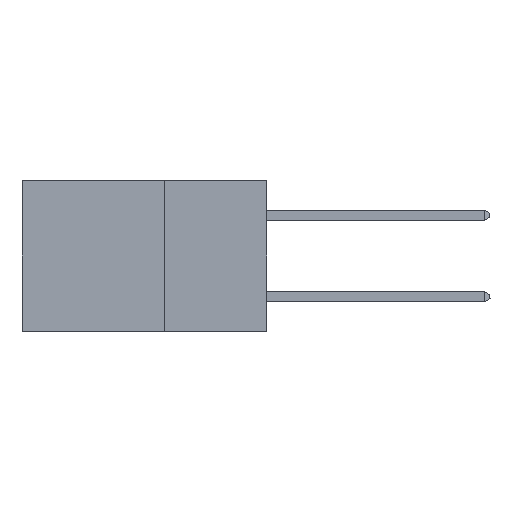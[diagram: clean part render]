
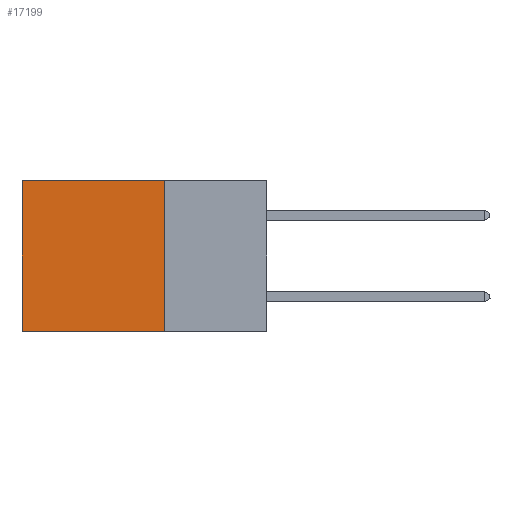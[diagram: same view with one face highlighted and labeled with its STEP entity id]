
A CAD part, left-side view. The second image highlights one B-rep face of the part: STEP entity #17199.
In plain terms, the highlighted planar face has unit normal (-1, 0, 0).
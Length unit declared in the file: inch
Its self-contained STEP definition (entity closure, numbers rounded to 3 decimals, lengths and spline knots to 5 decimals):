
#155 = VERTEX_POINT ( 'NONE', #15002 ) ;
#659 = AXIS2_PLACEMENT_3D ( 'NONE', #4516, #7272, #16826 ) ;
#1121 = EDGE_CURVE ( 'NONE', #13793, #7417, #9360, .T. ) ;
#1685 = ORIENTED_EDGE ( 'NONE', *, *, #1121, .F. ) ;
#1804 = CARTESIAN_POINT ( 'NONE',  ( 0.2875, 0.25, -0.37 ) ) ;
#2477 = VECTOR ( 'NONE', #17582, 39.37008 ) ;
#3450 = ORIENTED_EDGE ( 'NONE', *, *, #7479, .F. ) ;
#3462 = VECTOR ( 'NONE', #14534, 39.37008 ) ;
#4326 = EDGE_CURVE ( 'NONE', #155, #13900, #7535, .T. ) ;
#4461 = PLANE ( 'NONE',  #659 ) ;
#4516 = CARTESIAN_POINT ( 'NONE',  ( 0.2875, 0.25, 0. ) ) ;
#6009 = ORIENTED_EDGE ( 'NONE', *, *, #13868, .T. ) ;
#6353 = CARTESIAN_POINT ( 'NONE',  ( 0.2875, 0.25, 0. ) ) ;
#6378 = CARTESIAN_POINT ( 'NONE',  ( 0.2875, 0.6, 0. ) ) ;
#7272 = DIRECTION ( 'NONE',  ( 1., 0., 0. ) ) ;
#7417 = VERTEX_POINT ( 'NONE', #1804 ) ;
#7479 = EDGE_CURVE ( 'NONE', #7417, #13900, #15963, .T. ) ;
#7535 = LINE ( 'NONE', #6378, #3462 ) ;
#7591 = CARTESIAN_POINT ( 'NONE',  ( 0.2875, 0.25, 0. ) ) ;
#7642 = ORIENTED_EDGE ( 'NONE', *, *, #4326, .T. ) ;
#7858 = VECTOR ( 'NONE', #17076, 39.37008 ) ;
#8955 = VECTOR ( 'NONE', #13176, 39.37008 ) ;
#9360 = LINE ( 'NONE', #9853, #2477 ) ;
#9390 = LINE ( 'NONE', #6353, #8955 ) ;
#9853 = CARTESIAN_POINT ( 'NONE',  ( 0.2875, 0.25, 0. ) ) ;
#11206 = EDGE_LOOP ( 'NONE', ( #7642, #3450, #1685, #6009 ) ) ;
#11857 = CARTESIAN_POINT ( 'NONE',  ( 0.2875, 0.6, -0.37 ) ) ;
#13176 = DIRECTION ( 'NONE',  ( 0., 1., 0. ) ) ;
#13793 = VERTEX_POINT ( 'NONE', #7591 ) ;
#13868 = EDGE_CURVE ( 'NONE', #13793, #155, #9390, .T. ) ;
#13900 = VERTEX_POINT ( 'NONE', #11857 ) ;
#14202 = FACE_OUTER_BOUND ( 'NONE', #11206, .T. ) ;
#14534 = DIRECTION ( 'NONE',  ( 0., 0., -1. ) ) ;
#15002 = CARTESIAN_POINT ( 'NONE',  ( 0.2875, 0.6, 0. ) ) ;
#15689 = CARTESIAN_POINT ( 'NONE',  ( 0.2875, 0.25, -0.37 ) ) ;
#15963 = LINE ( 'NONE', #15689, #7858 ) ;
#16826 = DIRECTION ( 'NONE',  ( 0., 0., -1. ) ) ;
#17076 = DIRECTION ( 'NONE',  ( 0., 1., 0. ) ) ;
#17199 = ADVANCED_FACE ( 'NONE', ( #14202 ), #4461, .F. ) ;
#17582 = DIRECTION ( 'NONE',  ( 0., 0., -1. ) ) ;
